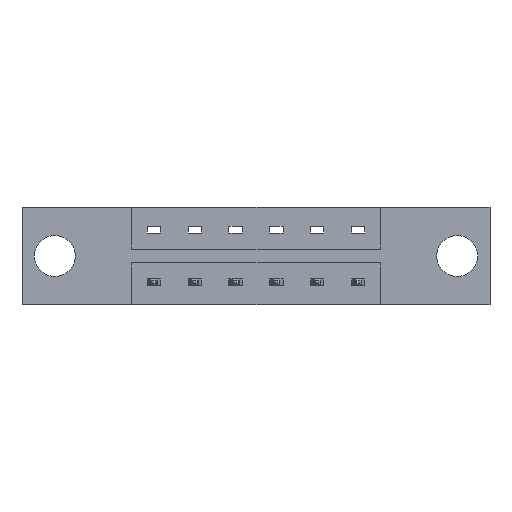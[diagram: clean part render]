
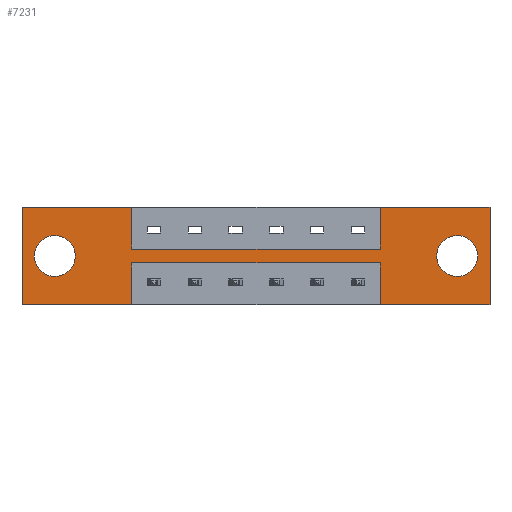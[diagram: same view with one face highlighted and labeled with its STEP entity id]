
A CAD part, front view. The second image highlights one B-rep face of the part: STEP entity #7231.
In plain terms, the highlighted planar face has unit normal (0, -1, 0).
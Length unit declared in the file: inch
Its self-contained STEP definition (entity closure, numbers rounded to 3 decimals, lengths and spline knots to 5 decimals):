
#79 = LINE ( 'NONE', #5316, #5229 ) ;
#87 = CARTESIAN_POINT ( 'NONE',  ( 1.659, 0., -0.107 ) ) ;
#125 = EDGE_CURVE ( 'NONE', #5681, #7263, #381, .T. ) ;
#134 = VERTEX_POINT ( 'NONE', #7270 ) ;
#339 = ORIENTED_EDGE ( 'NONE', *, *, #8138, .F. ) ;
#381 = LINE ( 'NONE', #2582, #2063 ) ;
#387 = ORIENTED_EDGE ( 'NONE', *, *, #2323, .F. ) ;
#531 = DIRECTION ( 'NONE',  ( 0., 0., -1. ) ) ;
#565 = DIRECTION ( 'NONE',  ( 0., 0., 1. ) ) ;
#574 = DIRECTION ( 'NONE',  ( 0., 1., 0. ) ) ;
#578 = CARTESIAN_POINT ( 'NONE',  ( 0.125, 0., -0.185 ) ) ;
#595 = CARTESIAN_POINT ( 'NONE',  ( 0.4175, 0., -0.1585 ) ) ;
#596 = FACE_OUTER_BOUND ( 'NONE', #5998, .T. ) ;
#700 = ORIENTED_EDGE ( 'NONE', *, *, #7855, .F. ) ;
#719 = ORIENTED_EDGE ( 'NONE', *, *, #1743, .F. ) ;
#908 = LINE ( 'NONE', #595, #5748 ) ;
#911 = VECTOR ( 'NONE', #2552, 39.37008 ) ;
#917 = ORIENTED_EDGE ( 'NONE', *, *, #3949, .F. ) ;
#1124 = EDGE_CURVE ( 'NONE', #3777, #4801, #5481, .T. ) ;
#1161 = VECTOR ( 'NONE', #3860, 39.37008 ) ;
#1174 = CARTESIAN_POINT ( 'NONE',  ( 0.4175, 0., -0.1585 ) ) ;
#1181 = ORIENTED_EDGE ( 'NONE', *, *, #3907, .F. ) ;
#1185 = ORIENTED_EDGE ( 'NONE', *, *, #4499, .T. ) ;
#1229 = CIRCLE ( 'NONE', #1265, 0.078 ) ;
#1265 = AXIS2_PLACEMENT_3D ( 'NONE', #578, #574, #565 ) ;
#1321 = VERTEX_POINT ( 'NONE', #5059 ) ;
#1334 = VECTOR ( 'NONE', #2173, 39.37008 ) ;
#1369 = LINE ( 'NONE', #7575, #911 ) ;
#1389 = CARTESIAN_POINT ( 'NONE',  ( 1.3665, 0., -0.1585 ) ) ;
#1427 = CARTESIAN_POINT ( 'NONE',  ( 1.784, 0., 0. ) ) ;
#1461 = CARTESIAN_POINT ( 'NONE',  ( 0.125, 0., -0.107 ) ) ;
#1491 = CARTESIAN_POINT ( 'NONE',  ( 1.3665, 0., -0.1585 ) ) ;
#1494 = CARTESIAN_POINT ( 'NONE',  ( 0., 0., -0.37 ) ) ;
#1500 = DIRECTION ( 'NONE',  ( 0., 0., 1. ) ) ;
#1541 = ORIENTED_EDGE ( 'NONE', *, *, #5914, .F. ) ;
#1661 = VERTEX_POINT ( 'NONE', #3208 ) ;
#1674 = EDGE_CURVE ( 'NONE', #1841, #1661, #2239, .T. ) ;
#1676 = DIRECTION ( 'NONE',  ( -1., 0., 0. ) ) ;
#1717 = ORIENTED_EDGE ( 'NONE', *, *, #5514, .F. ) ;
#1743 = EDGE_CURVE ( 'NONE', #3302, #5681, #2967, .T. ) ;
#1841 = VERTEX_POINT ( 'NONE', #87 ) ;
#1938 = ORIENTED_EDGE ( 'NONE', *, *, #125, .F. ) ;
#1963 = VECTOR ( 'NONE', #1500, 39.37008 ) ;
#1985 = ORIENTED_EDGE ( 'NONE', *, *, #1674, .T. ) ;
#2063 = VECTOR ( 'NONE', #6629, 39.37008 ) ;
#2173 = DIRECTION ( 'NONE',  ( 1., 0., 0. ) ) ;
#2205 = DIRECTION ( 'NONE',  ( 0., 1., 0. ) ) ;
#2222 = VERTEX_POINT ( 'NONE', #1174 ) ;
#2239 = CIRCLE ( 'NONE', #2334, 0.078 ) ;
#2323 = EDGE_CURVE ( 'NONE', #8160, #2222, #908, .T. ) ;
#2334 = AXIS2_PLACEMENT_3D ( 'NONE', #4463, #7331, #7703 ) ;
#2356 = ORIENTED_EDGE ( 'NONE', *, *, #3810, .T. ) ;
#2396 = CARTESIAN_POINT ( 'NONE',  ( 0., 0., 0. ) ) ;
#2433 = VECTOR ( 'NONE', #2849, 39.37008 ) ;
#2454 = FACE_BOUND ( 'NONE', #6962, .T. ) ;
#2511 = CARTESIAN_POINT ( 'NONE',  ( 0.4175, 0., -0.2115 ) ) ;
#2552 = DIRECTION ( 'NONE',  ( 1., 0., 0. ) ) ;
#2582 = CARTESIAN_POINT ( 'NONE',  ( 0.4175, 0., -0.2115 ) ) ;
#2585 = DIRECTION ( 'NONE',  ( 1., 0., 0. ) ) ;
#2828 = LINE ( 'NONE', #1427, #6204 ) ;
#2849 = DIRECTION ( 'NONE',  ( 0., 0., 1. ) ) ;
#2871 = CARTESIAN_POINT ( 'NONE',  ( 0.4175, 0., 0. ) ) ;
#2959 = CARTESIAN_POINT ( 'NONE',  ( 1.784, 0., 0. ) ) ;
#2967 = LINE ( 'NONE', #4671, #1161 ) ;
#2972 = DIRECTION ( 'NONE',  ( 0., 0., -1. ) ) ;
#3053 = DIRECTION ( 'NONE',  ( 0., -1., 0. ) ) ;
#3078 = CARTESIAN_POINT ( 'NONE',  ( 0., 0., -0.37 ) ) ;
#3115 = LINE ( 'NONE', #2396, #1334 ) ;
#3208 = CARTESIAN_POINT ( 'NONE',  ( 1.659, 0., -0.263 ) ) ;
#3229 = VERTEX_POINT ( 'NONE', #6327 ) ;
#3267 = PLANE ( 'NONE',  #4283 ) ;
#3302 = VERTEX_POINT ( 'NONE', #6198 ) ;
#3303 = CARTESIAN_POINT ( 'NONE',  ( 0.4175, 0., -0.1585 ) ) ;
#3477 = CARTESIAN_POINT ( 'NONE',  ( 0., 0., 0. ) ) ;
#3529 = CARTESIAN_POINT ( 'NONE',  ( 1.3665, 0., -0.2115 ) ) ;
#3549 = CARTESIAN_POINT ( 'NONE',  ( 0.125, 0., -0.185 ) ) ;
#3555 = LINE ( 'NONE', #7994, #5073 ) ;
#3633 = DIRECTION ( 'NONE',  ( 0., 0., 1. ) ) ;
#3683 = LINE ( 'NONE', #1491, #1963 ) ;
#3753 = VECTOR ( 'NONE', #1676, 39.37008 ) ;
#3777 = VERTEX_POINT ( 'NONE', #4164 ) ;
#3810 = EDGE_CURVE ( 'NONE', #7525, #134, #5813, .T. ) ;
#3860 = DIRECTION ( 'NONE',  ( 0., 0., 1. ) ) ;
#3907 = EDGE_CURVE ( 'NONE', #2222, #5923, #6703, .T. ) ;
#3948 = LINE ( 'NONE', #3477, #2433 ) ;
#3949 = EDGE_CURVE ( 'NONE', #1321, #4981, #3115, .T. ) ;
#4091 = ORIENTED_EDGE ( 'NONE', *, *, #4269, .F. ) ;
#4164 = CARTESIAN_POINT ( 'NONE',  ( 0.4175, 0., -0.37 ) ) ;
#4233 = ORIENTED_EDGE ( 'NONE', *, *, #8144, .T. ) ;
#4269 = EDGE_CURVE ( 'NONE', #4981, #8171, #2828, .T. ) ;
#4283 = AXIS2_PLACEMENT_3D ( 'NONE', #3078, #3053, #2972 ) ;
#4463 = CARTESIAN_POINT ( 'NONE',  ( 1.659, 0., -0.185 ) ) ;
#4499 = EDGE_CURVE ( 'NONE', #134, #7525, #1229, .T. ) ;
#4671 = CARTESIAN_POINT ( 'NONE',  ( 1.3665, 0., -0.2115 ) ) ;
#4801 = VERTEX_POINT ( 'NONE', #7771 ) ;
#4953 = DIRECTION ( 'NONE',  ( -1., 0., 0. ) ) ;
#4981 = VERTEX_POINT ( 'NONE', #2959 ) ;
#5025 = VECTOR ( 'NONE', #2585, 39.37008 ) ;
#5059 = CARTESIAN_POINT ( 'NONE',  ( 1.3665, 0., 0. ) ) ;
#5073 = VECTOR ( 'NONE', #4953, 39.37008 ) ;
#5229 = VECTOR ( 'NONE', #5324, 39.37008 ) ;
#5316 = CARTESIAN_POINT ( 'NONE',  ( 0.4175, 0., -0.2115 ) ) ;
#5324 = DIRECTION ( 'NONE',  ( 0., 0., -1. ) ) ;
#5481 = LINE ( 'NONE', #1494, #3753 ) ;
#5514 = EDGE_CURVE ( 'NONE', #7263, #3777, #79, .T. ) ;
#5579 = ORIENTED_EDGE ( 'NONE', *, *, #7720, .F. ) ;
#5681 = VERTEX_POINT ( 'NONE', #3529 ) ;
#5748 = VECTOR ( 'NONE', #8020, 39.37008 ) ;
#5813 = CIRCLE ( 'NONE', #6109, 0.078 ) ;
#5855 = FACE_BOUND ( 'NONE', #8245, .T. ) ;
#5914 = EDGE_CURVE ( 'NONE', #5923, #1321, #3683, .T. ) ;
#5923 = VERTEX_POINT ( 'NONE', #1389 ) ;
#5998 = EDGE_LOOP ( 'NONE', ( #719, #5579, #4091, #917, #1541, #1181, #387, #700, #339, #6757, #1717, #1938 ) ) ;
#6048 = CARTESIAN_POINT ( 'NONE',  ( 1.659, 0., -0.185 ) ) ;
#6075 = CARTESIAN_POINT ( 'NONE',  ( 1.784, 0., -0.37 ) ) ;
#6109 = AXIS2_PLACEMENT_3D ( 'NONE', #3549, #8145, #3633 ) ;
#6198 = CARTESIAN_POINT ( 'NONE',  ( 1.3665, 0., -0.37 ) ) ;
#6204 = VECTOR ( 'NONE', #531, 39.37008 ) ;
#6327 = CARTESIAN_POINT ( 'NONE',  ( 0., 0., 0. ) ) ;
#6629 = DIRECTION ( 'NONE',  ( -1., 0., 0. ) ) ;
#6680 = DIRECTION ( 'NONE',  ( 0., 0., -1. ) ) ;
#6703 = LINE ( 'NONE', #3303, #5025 ) ;
#6757 = ORIENTED_EDGE ( 'NONE', *, *, #1124, .F. ) ;
#6962 = EDGE_LOOP ( 'NONE', ( #1985, #4233 ) ) ;
#7103 = CIRCLE ( 'NONE', #7169, 0.078 ) ;
#7169 = AXIS2_PLACEMENT_3D ( 'NONE', #6048, #2205, #6680 ) ;
#7231 = ADVANCED_FACE ( 'NONE', ( #2454, #5855, #596 ), #3267, .T. ) ;
#7263 = VERTEX_POINT ( 'NONE', #2511 ) ;
#7270 = CARTESIAN_POINT ( 'NONE',  ( 0.125, 0., -0.263 ) ) ;
#7331 = DIRECTION ( 'NONE',  ( 0., 1., 0. ) ) ;
#7525 = VERTEX_POINT ( 'NONE', #1461 ) ;
#7575 = CARTESIAN_POINT ( 'NONE',  ( 0., 0., 0. ) ) ;
#7703 = DIRECTION ( 'NONE',  ( 0., 0., -1. ) ) ;
#7720 = EDGE_CURVE ( 'NONE', #8171, #3302, #3555, .T. ) ;
#7771 = CARTESIAN_POINT ( 'NONE',  ( 0., 0., -0.37 ) ) ;
#7855 = EDGE_CURVE ( 'NONE', #3229, #8160, #1369, .T. ) ;
#7994 = CARTESIAN_POINT ( 'NONE',  ( 0., 0., -0.37 ) ) ;
#8020 = DIRECTION ( 'NONE',  ( 0., 0., -1. ) ) ;
#8138 = EDGE_CURVE ( 'NONE', #4801, #3229, #3948, .T. ) ;
#8144 = EDGE_CURVE ( 'NONE', #1661, #1841, #7103, .T. ) ;
#8145 = DIRECTION ( 'NONE',  ( 0., 1., 0. ) ) ;
#8160 = VERTEX_POINT ( 'NONE', #2871 ) ;
#8171 = VERTEX_POINT ( 'NONE', #6075 ) ;
#8245 = EDGE_LOOP ( 'NONE', ( #2356, #1185 ) ) ;
